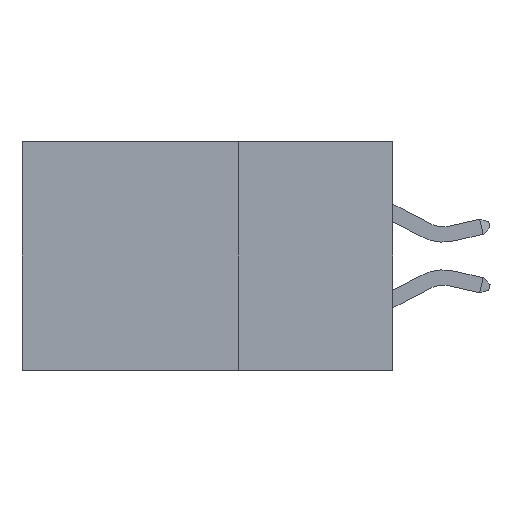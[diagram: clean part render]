
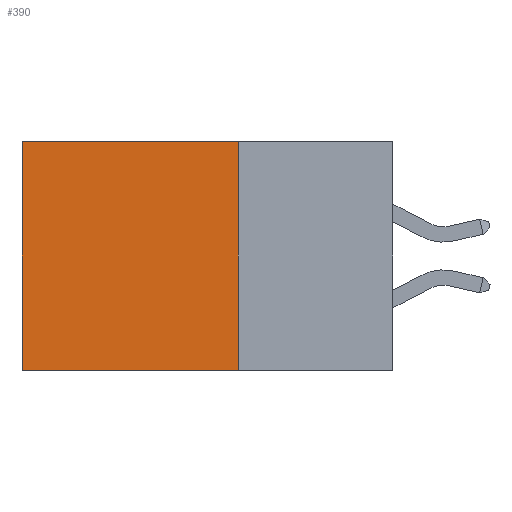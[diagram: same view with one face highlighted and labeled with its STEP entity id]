
A CAD part, left-side view. The second image highlights one B-rep face of the part: STEP entity #390.
In plain terms, the highlighted planar face has unit normal (-1, 0, 0).
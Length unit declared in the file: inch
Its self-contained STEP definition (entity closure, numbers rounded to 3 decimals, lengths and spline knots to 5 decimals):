
#390 = ADVANCED_FACE ( 'NONE', ( #611 ), #2870, .F. ) ;
#556 = CARTESIAN_POINT ( 'NONE',  ( 0.2875, 0.25, 0. ) ) ;
#611 = FACE_OUTER_BOUND ( 'NONE', #12535, .T. ) ;
#697 = AXIS2_PLACEMENT_3D ( 'NONE', #2521, #2856, #4483 ) ;
#957 = VERTEX_POINT ( 'NONE', #10598 ) ;
#1132 = EDGE_CURVE ( 'NONE', #6172, #10333, #7598, .T. ) ;
#2050 = VECTOR ( 'NONE', #2431, 39.37008 ) ;
#2217 = ORIENTED_EDGE ( 'NONE', *, *, #1132, .T. ) ;
#2431 = DIRECTION ( 'NONE',  ( 0., 0., -1. ) ) ;
#2521 = CARTESIAN_POINT ( 'NONE',  ( 0.2875, 0.25, 0. ) ) ;
#2633 = ORIENTED_EDGE ( 'NONE', *, *, #2686, .F. ) ;
#2686 = EDGE_CURVE ( 'NONE', #957, #3372, #6290, .T. ) ;
#2856 = DIRECTION ( 'NONE',  ( 1., 0., 0. ) ) ;
#2870 = PLANE ( 'NONE',  #697 ) ;
#3044 = CARTESIAN_POINT ( 'NONE',  ( 0.2875, 0.6, -0.37 ) ) ;
#3071 = VECTOR ( 'NONE', #6156, 39.37008 ) ;
#3372 = VERTEX_POINT ( 'NONE', #9109 ) ;
#3737 = LINE ( 'NONE', #12819, #3071 ) ;
#4120 = CARTESIAN_POINT ( 'NONE',  ( 0.2875, 0.6, 0. ) ) ;
#4483 = DIRECTION ( 'NONE',  ( 0., 0., -1. ) ) ;
#4514 = CARTESIAN_POINT ( 'NONE',  ( 0.2875, 0.6, 0. ) ) ;
#5826 = DIRECTION ( 'NONE',  ( 0., 0., -1. ) ) ;
#5919 = LINE ( 'NONE', #556, #6207 ) ;
#6156 = DIRECTION ( 'NONE',  ( 0., 1., 0. ) ) ;
#6172 = VERTEX_POINT ( 'NONE', #4120 ) ;
#6207 = VECTOR ( 'NONE', #12610, 39.37008 ) ;
#6290 = LINE ( 'NONE', #7569, #11437 ) ;
#6713 = ORIENTED_EDGE ( 'NONE', *, *, #10203, .T. ) ;
#7569 = CARTESIAN_POINT ( 'NONE',  ( 0.2875, 0.25, 0. ) ) ;
#7598 = LINE ( 'NONE', #4514, #2050 ) ;
#9109 = CARTESIAN_POINT ( 'NONE',  ( 0.2875, 0.25, -0.37 ) ) ;
#10203 = EDGE_CURVE ( 'NONE', #957, #6172, #5919, .T. ) ;
#10333 = VERTEX_POINT ( 'NONE', #3044 ) ;
#10598 = CARTESIAN_POINT ( 'NONE',  ( 0.2875, 0.25, 0. ) ) ;
#11437 = VECTOR ( 'NONE', #5826, 39.37008 ) ;
#11511 = ORIENTED_EDGE ( 'NONE', *, *, #12169, .F. ) ;
#12169 = EDGE_CURVE ( 'NONE', #3372, #10333, #3737, .T. ) ;
#12535 = EDGE_LOOP ( 'NONE', ( #2217, #11511, #2633, #6713 ) ) ;
#12610 = DIRECTION ( 'NONE',  ( 0., 1., 0. ) ) ;
#12819 = CARTESIAN_POINT ( 'NONE',  ( 0.2875, 0.25, -0.37 ) ) ;
